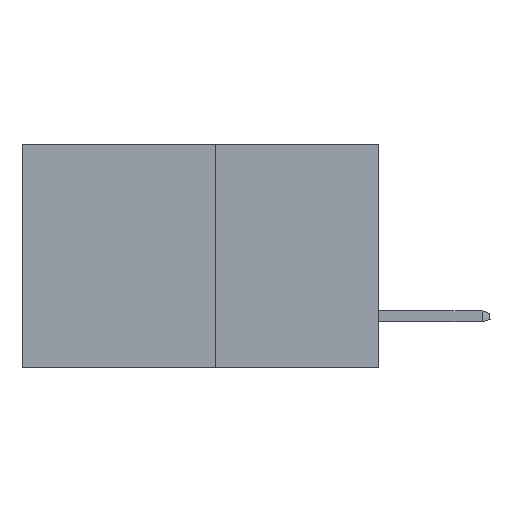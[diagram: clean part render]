
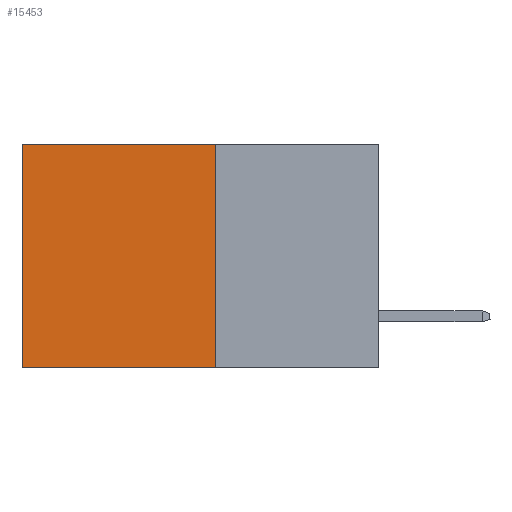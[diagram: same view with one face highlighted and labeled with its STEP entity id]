
A CAD part, left-side view. The second image highlights one B-rep face of the part: STEP entity #15453.
In plain terms, the highlighted planar face has unit normal (-1, 0, 0).
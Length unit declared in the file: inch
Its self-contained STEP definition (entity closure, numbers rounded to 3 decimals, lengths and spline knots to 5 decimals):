
#207 = EDGE_CURVE ( 'NONE', #668, #12278, #7941, .T. ) ;
#240 = VECTOR ( 'NONE', #9253, 39.37008 ) ;
#483 = VERTEX_POINT ( 'NONE', #15240 ) ;
#668 = VERTEX_POINT ( 'NONE', #3561 ) ;
#971 = VECTOR ( 'NONE', #4654, 39.37008 ) ;
#1326 = VECTOR ( 'NONE', #4139, 39.37008 ) ;
#2572 = ORIENTED_EDGE ( 'NONE', *, *, #16129, .T. ) ;
#2735 = PLANE ( 'NONE',  #9737 ) ;
#3207 = FACE_OUTER_BOUND ( 'NONE', #12626, .T. ) ;
#3561 = CARTESIAN_POINT ( 'NONE',  ( 0.277, 0.27, 0. ) ) ;
#3753 = EDGE_CURVE ( 'NONE', #668, #483, #5734, .T. ) ;
#4100 = DIRECTION ( 'NONE',  ( 1., 0., 0. ) ) ;
#4139 = DIRECTION ( 'NONE',  ( 0., 0., -1. ) ) ;
#4654 = DIRECTION ( 'NONE',  ( 0., 1., 0. ) ) ;
#4952 = CARTESIAN_POINT ( 'NONE',  ( 0.277, 0.59, -0.37 ) ) ;
#5405 = CARTESIAN_POINT ( 'NONE',  ( 0.277, 0.27, -0.37 ) ) ;
#5734 = LINE ( 'NONE', #5405, #15701 ) ;
#7939 = CARTESIAN_POINT ( 'NONE',  ( 0.277, 0.27, -0.37 ) ) ;
#7941 = LINE ( 'NONE', #15282, #971 ) ;
#8945 = ORIENTED_EDGE ( 'NONE', *, *, #207, .T. ) ;
#9094 = CARTESIAN_POINT ( 'NONE',  ( 0.277, 0.59, 0. ) ) ;
#9253 = DIRECTION ( 'NONE',  ( 0., 1., 0. ) ) ;
#9737 = AXIS2_PLACEMENT_3D ( 'NONE', #11889, #4100, #13242 ) ;
#11128 = LINE ( 'NONE', #7939, #240 ) ;
#11198 = EDGE_CURVE ( 'NONE', #483, #16468, #11128, .T. ) ;
#11802 = LINE ( 'NONE', #14614, #1326 ) ;
#11815 = ORIENTED_EDGE ( 'NONE', *, *, #3753, .F. ) ;
#11889 = CARTESIAN_POINT ( 'NONE',  ( 0.277, 0.27, -0.37 ) ) ;
#12278 = VERTEX_POINT ( 'NONE', #9094 ) ;
#12626 = EDGE_LOOP ( 'NONE', ( #2572, #13472, #11815, #8945 ) ) ;
#13138 = DIRECTION ( 'NONE',  ( 0., 0., -1. ) ) ;
#13242 = DIRECTION ( 'NONE',  ( 0., 0., -1. ) ) ;
#13472 = ORIENTED_EDGE ( 'NONE', *, *, #11198, .F. ) ;
#14614 = CARTESIAN_POINT ( 'NONE',  ( 0.277, 0.59, -0.37 ) ) ;
#15240 = CARTESIAN_POINT ( 'NONE',  ( 0.277, 0.27, -0.37 ) ) ;
#15282 = CARTESIAN_POINT ( 'NONE',  ( 0.277, 0.27, 0. ) ) ;
#15453 = ADVANCED_FACE ( 'NONE', ( #3207 ), #2735, .F. ) ;
#15701 = VECTOR ( 'NONE', #13138, 39.37008 ) ;
#16129 = EDGE_CURVE ( 'NONE', #12278, #16468, #11802, .T. ) ;
#16468 = VERTEX_POINT ( 'NONE', #4952 ) ;
